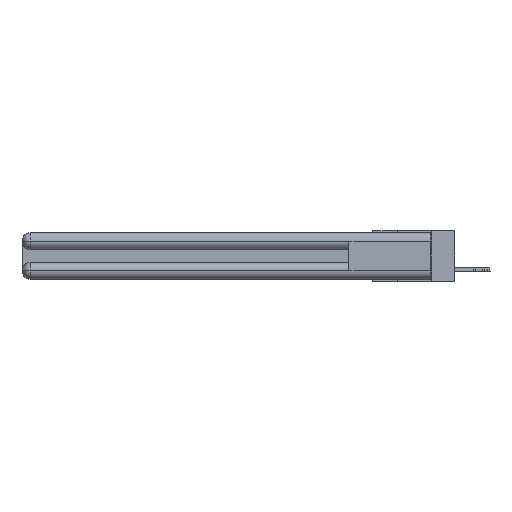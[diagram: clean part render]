
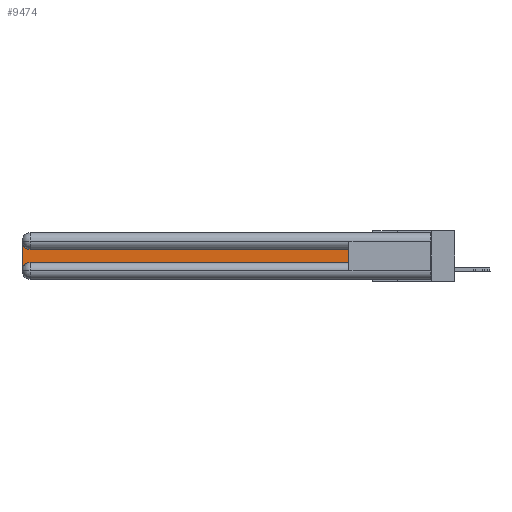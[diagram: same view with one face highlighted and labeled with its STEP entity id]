
A CAD part, left-side view. The second image highlights one B-rep face of the part: STEP entity #9474.
In plain terms, the highlighted planar face has unit normal (-1, 0, 0).
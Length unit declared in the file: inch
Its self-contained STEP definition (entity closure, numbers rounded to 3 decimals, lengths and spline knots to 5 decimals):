
#5 = LINE ( 'NONE', #86, #12626 ) ;
#86 = CARTESIAN_POINT ( 'NONE',  ( 0.075, 3., -0.2175 ) ) ;
#1223 = LINE ( 'NONE', #3757, #2323 ) ;
#1916 = ORIENTED_EDGE ( 'NONE', *, *, #25714, .T. ) ;
#2323 = VECTOR ( 'NONE', #17366, 39.37008 ) ;
#2580 = VECTOR ( 'NONE', #3839, 39.37008 ) ;
#2766 = CARTESIAN_POINT ( 'NONE',  ( 0.075, 0.6, -0.2175 ) ) ;
#3757 = CARTESIAN_POINT ( 'NONE',  ( 0.075, 0.6, -0.1225 ) ) ;
#3839 = DIRECTION ( 'NONE',  ( 0., -1., 0. ) ) ;
#4400 = DIRECTION ( 'NONE',  ( 1., 0., 0. ) ) ;
#4404 = VERTEX_POINT ( 'NONE', #5298 ) ;
#4551 = EDGE_CURVE ( 'NONE', #13032, #20128, #1223, .T. ) ;
#5298 = CARTESIAN_POINT ( 'NONE',  ( 0.075, 3., -0.2775 ) ) ;
#5299 = VERTEX_POINT ( 'NONE', #2766 ) ;
#6077 = CARTESIAN_POINT ( 'NONE',  ( 0.075, 2.94, -0.1225 ) ) ;
#6794 = EDGE_LOOP ( 'NONE', ( #27605, #16290, #7691, #27229, #12689, #1916 ) ) ;
#7691 = ORIENTED_EDGE ( 'NONE', *, *, #9378, .T. ) ;
#9378 = EDGE_CURVE ( 'NONE', #9520, #4404, #5, .T. ) ;
#9474 = ADVANCED_FACE ( 'NONE', ( #20006 ), #24574, .F. ) ;
#9520 = VERTEX_POINT ( 'NONE', #10327 ) ;
#10059 = CIRCLE ( 'NONE', #14108, 0.06 ) ;
#10266 = LINE ( 'NONE', #14899, #2580 ) ;
#10327 = CARTESIAN_POINT ( 'NONE',  ( 0.075, 3., -0.0625 ) ) ;
#11220 = LINE ( 'NONE', #14958, #14743 ) ;
#12626 = VECTOR ( 'NONE', #27616, 39.37008 ) ;
#12689 = ORIENTED_EDGE ( 'NONE', *, *, #17561, .T. ) ;
#13032 = VERTEX_POINT ( 'NONE', #16253 ) ;
#13293 = CARTESIAN_POINT ( 'NONE',  ( 0.075, 3., -0.1225 ) ) ;
#13699 = CARTESIAN_POINT ( 'NONE',  ( 0.075, 2.94, -0.2175 ) ) ;
#13949 = DIRECTION ( 'NONE',  ( 0., 0., 1. ) ) ;
#14108 = AXIS2_PLACEMENT_3D ( 'NONE', #14468, #23313, #16340 ) ;
#14468 = CARTESIAN_POINT ( 'NONE',  ( 0.075, 2.94, -0.0625 ) ) ;
#14743 = VECTOR ( 'NONE', #13949, 39.37008 ) ;
#14899 = CARTESIAN_POINT ( 'NONE',  ( 0.075, 0.6, -0.2175 ) ) ;
#14958 = CARTESIAN_POINT ( 'NONE',  ( 0.075, 0.6, -0.2175 ) ) ;
#15018 = VERTEX_POINT ( 'NONE', #13699 ) ;
#15079 = AXIS2_PLACEMENT_3D ( 'NONE', #26818, #4400, #18031 ) ;
#15080 = EDGE_CURVE ( 'NONE', #20128, #9520, #10059, .T. ) ;
#16253 = CARTESIAN_POINT ( 'NONE',  ( 0.075, 0.6, -0.1225 ) ) ;
#16290 = ORIENTED_EDGE ( 'NONE', *, *, #15080, .T. ) ;
#16340 = DIRECTION ( 'NONE',  ( 0., 0., -1. ) ) ;
#17366 = DIRECTION ( 'NONE',  ( 0., 1., 0. ) ) ;
#17561 = EDGE_CURVE ( 'NONE', #15018, #5299, #10266, .T. ) ;
#18031 = DIRECTION ( 'NONE',  ( 0., 0., -1. ) ) ;
#20006 = FACE_OUTER_BOUND ( 'NONE', #6794, .T. ) ;
#20128 = VERTEX_POINT ( 'NONE', #6077 ) ;
#22239 = DIRECTION ( 'NONE',  ( 0., 0., -1. ) ) ;
#23313 = DIRECTION ( 'NONE',  ( 1., 0., 0. ) ) ;
#24017 = AXIS2_PLACEMENT_3D ( 'NONE', #13293, #26439, #22239 ) ;
#24574 = PLANE ( 'NONE',  #24017 ) ;
#25553 = CIRCLE ( 'NONE', #15079, 0.06 ) ;
#25714 = EDGE_CURVE ( 'NONE', #5299, #13032, #11220, .T. ) ;
#26439 = DIRECTION ( 'NONE',  ( 1., 0., 0. ) ) ;
#26607 = EDGE_CURVE ( 'NONE', #4404, #15018, #25553, .T. ) ;
#26818 = CARTESIAN_POINT ( 'NONE',  ( 0.075, 2.94, -0.2775 ) ) ;
#27229 = ORIENTED_EDGE ( 'NONE', *, *, #26607, .T. ) ;
#27605 = ORIENTED_EDGE ( 'NONE', *, *, #4551, .T. ) ;
#27616 = DIRECTION ( 'NONE',  ( 0., 0., -1. ) ) ;
